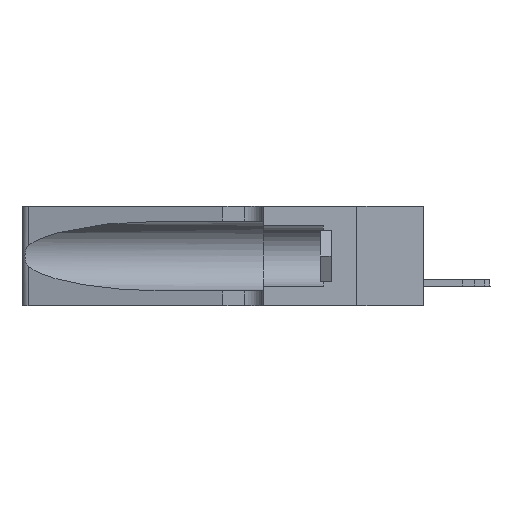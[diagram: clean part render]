
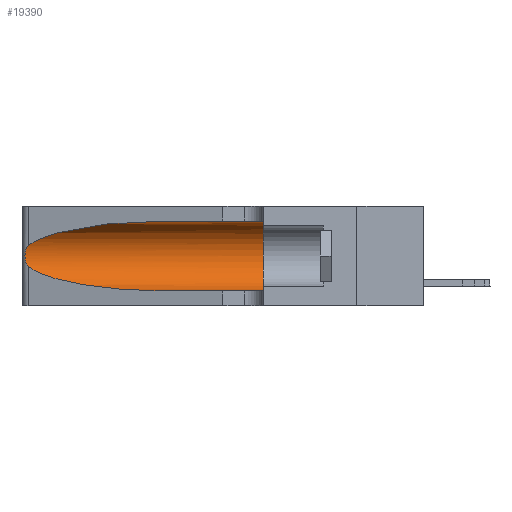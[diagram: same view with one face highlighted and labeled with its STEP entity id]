
A CAD part, left-side view. The second image highlights one B-rep face of the part: STEP entity #19390.
In plain terms, the highlighted cylindrical face has radius 3.308 mm (diameter 6.617 mm), a partial arc.
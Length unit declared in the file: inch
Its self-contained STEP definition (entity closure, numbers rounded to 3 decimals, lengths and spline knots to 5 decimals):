
#1160 = EDGE_CURVE ( 'NONE', #10669, #20331, #22495, .T. ) ;
#1210 = CARTESIAN_POINT ( 'NONE',  ( 0.25487, 1.22718, 0.22369 ) ) ;
#1453 = VERTEX_POINT ( 'NONE', #5880 ) ;
#1458 = AXIS2_PLACEMENT_3D ( 'NONE', #6180, #21093, #14717 ) ;
#3274 = CARTESIAN_POINT ( 'NONE',  ( 0.1305, 1.61858, 0.31525 ) ) ;
#3542 = CARTESIAN_POINT ( 'NONE',  ( 0.1305, 1.61858, 0.05475 ) ) ;
#3585 =( BOUNDED_CURVE ( )  B_SPLINE_CURVE ( 3, ( #24011, #21808, #19467, #15266 ),
 .UNSPECIFIED., .F., .F. ) 
 B_SPLINE_CURVE_WITH_KNOTS ( ( 4, 4 ),
 ( 3.44316, 4.71239 ),
 .UNSPECIFIED. ) 
 CURVE ( )  GEOMETRIC_REPRESENTATION_ITEM ( )  RATIONAL_B_SPLINE_CURVE ( ( 1., 0.87, 0.87, 1. ) ) 
 REPRESENTATION_ITEM ( '' )  );
#4098 = CYLINDRICAL_SURFACE ( 'NONE', #4486, 0.13025 ) ;
#4153 = LINE ( 'NONE', #3274, #22748 ) ;
#4486 = AXIS2_PLACEMENT_3D ( 'NONE', #14302, #27148, #7990 ) ;
#4763 = FACE_OUTER_BOUND ( 'NONE', #14168, .T. ) ;
#4936 = CARTESIAN_POINT ( 'NONE',  ( 0.1305, 0.72297, 0.31525 ) ) ;
#5878 = CARTESIAN_POINT ( 'NONE',  ( 0.26075, 1.23896, 0.178 ) ) ;
#5880 = CARTESIAN_POINT ( 'NONE',  ( 0.1305, 0.35, 0.05475 ) ) ;
#5947 = B_SPLINE_CURVE_WITH_KNOTS ( 'NONE', 3,
 ( #18509, #6045, #10028, #24920, #16462, #18599, #12280, #5878, #20768, #12462, #10219, #12368, #20968, #7999 ),
 .UNSPECIFIED., .F., .F.,
 ( 4, 2, 2, 2, 2, 2, 4 ),
 ( 0., 0.00027, 0.00053, 0.00107, 0.0016, 0.00187, 0.00214 ),
 .UNSPECIFIED. ) ;
#6045 = CARTESIAN_POINT ( 'NONE',  ( 0.25555, 1.22994, 0.2215 ) ) ;
#6071 = ORIENTED_EDGE ( 'NONE', *, *, #1160, .T. ) ;
#6139 = CARTESIAN_POINT ( 'NONE',  ( 0.1305, 0.35, 0.31525 ) ) ;
#6180 = CARTESIAN_POINT ( 'NONE',  ( 0.1305, 0.35, 0.185 ) ) ;
#7990 = DIRECTION ( 'NONE',  ( 0., 0., -1. ) ) ;
#7999 = CARTESIAN_POINT ( 'NONE',  ( 0.25487, 1.22718, 0.14631 ) ) ;
#8107 = CARTESIAN_POINT ( 'NONE',  ( 0.18966, 0.96281, 0.31525 ) ) ;
#8493 = ORIENTED_EDGE ( 'NONE', *, *, #20028, .T. ) ;
#9845 = ORIENTED_EDGE ( 'NONE', *, *, #16774, .T. ) ;
#10028 = CARTESIAN_POINT ( 'NONE',  ( 0.25639, 1.23184, 0.21858 ) ) ;
#10219 = CARTESIAN_POINT ( 'NONE',  ( 0.25789, 1.23486, 0.15765 ) ) ;
#10669 = VERTEX_POINT ( 'NONE', #4936 ) ;
#11089 = VERTEX_POINT ( 'NONE', #26609 ) ;
#11314 = VERTEX_POINT ( 'NONE', #6139 ) ;
#11347 = ORIENTED_EDGE ( 'NONE', *, *, #13831, .T. ) ;
#12111 = VERTEX_POINT ( 'NONE', #17732 ) ;
#12280 = CARTESIAN_POINT ( 'NONE',  ( 0.26075, 1.23896, 0.19203 ) ) ;
#12368 = CARTESIAN_POINT ( 'NONE',  ( 0.25639, 1.23186, 0.15144 ) ) ;
#12462 = CARTESIAN_POINT ( 'NONE',  ( 0.25856, 1.23593, 0.16098 ) ) ;
#13447 = EDGE_CURVE ( 'NONE', #10669, #11314, #4153, .T. ) ;
#13667 = VECTOR ( 'NONE', #24621, 39.37008 ) ;
#13831 = EDGE_CURVE ( 'NONE', #11089, #12111, #3585, .T. ) ;
#14168 = EDGE_LOOP ( 'NONE', ( #6071, #9845, #11347, #8493, #18073, #17289 ) ) ;
#14302 = CARTESIAN_POINT ( 'NONE',  ( 0.1305, 1.61858, 0.185 ) ) ;
#14717 = DIRECTION ( 'NONE',  ( 0., 0., 1. ) ) ;
#15266 = CARTESIAN_POINT ( 'NONE',  ( 0.1305, 0.72297, 0.05475 ) ) ;
#16253 = EDGE_CURVE ( 'NONE', #11314, #1453, #23301, .T. ) ;
#16462 = CARTESIAN_POINT ( 'NONE',  ( 0.25854, 1.2359, 0.20912 ) ) ;
#16753 = CARTESIAN_POINT ( 'NONE',  ( 0.2373, 1.15595, 0.28018 ) ) ;
#16774 = EDGE_CURVE ( 'NONE', #20331, #11089, #5947, .T. ) ;
#17289 = ORIENTED_EDGE ( 'NONE', *, *, #13447, .F. ) ;
#17732 = CARTESIAN_POINT ( 'NONE',  ( 0.1305, 0.72297, 0.05475 ) ) ;
#17854 = DIRECTION ( 'NONE',  ( 0., -1., 0. ) ) ;
#18073 = ORIENTED_EDGE ( 'NONE', *, *, #16253, .F. ) ;
#18509 = CARTESIAN_POINT ( 'NONE',  ( 0.25487, 1.22718, 0.22369 ) ) ;
#18599 = CARTESIAN_POINT ( 'NONE',  ( 0.26018, 1.23835, 0.19895 ) ) ;
#19390 = ADVANCED_FACE ( 'NONE', ( #4763 ), #4098, .F. ) ;
#19467 = CARTESIAN_POINT ( 'NONE',  ( 0.18966, 0.96281, 0.05475 ) ) ;
#20019 = LINE ( 'NONE', #3542, #13667 ) ;
#20028 = EDGE_CURVE ( 'NONE', #12111, #1453, #20019, .T. ) ;
#20331 = VERTEX_POINT ( 'NONE', #1210 ) ;
#20768 = CARTESIAN_POINT ( 'NONE',  ( 0.26017, 1.23833, 0.17102 ) ) ;
#20887 = CARTESIAN_POINT ( 'NONE',  ( 0.1305, 0.72297, 0.31525 ) ) ;
#20968 = CARTESIAN_POINT ( 'NONE',  ( 0.25555, 1.22993, 0.14849 ) ) ;
#21093 = DIRECTION ( 'NONE',  ( 0., 1., 0. ) ) ;
#21808 = CARTESIAN_POINT ( 'NONE',  ( 0.2373, 1.15595, 0.08982 ) ) ;
#22495 =( BOUNDED_CURVE ( )  B_SPLINE_CURVE ( 3, ( #20887, #8107, #16753, #22994 ),
 .UNSPECIFIED., .F., .F. ) 
 B_SPLINE_CURVE_WITH_KNOTS ( ( 4, 4 ),
 ( 1.5708, 2.84003 ),
 .UNSPECIFIED. ) 
 CURVE ( )  GEOMETRIC_REPRESENTATION_ITEM ( )  RATIONAL_B_SPLINE_CURVE ( ( 1., 0.87, 0.87, 1. ) ) 
 REPRESENTATION_ITEM ( '' )  );
#22748 = VECTOR ( 'NONE', #17854, 39.37008 ) ;
#22994 = CARTESIAN_POINT ( 'NONE',  ( 0.25487, 1.22718, 0.22369 ) ) ;
#23301 = CIRCLE ( 'NONE', #1458, 0.13025 ) ;
#24011 = CARTESIAN_POINT ( 'NONE',  ( 0.25487, 1.22718, 0.14631 ) ) ;
#24621 = DIRECTION ( 'NONE',  ( 0., -1., 0. ) ) ;
#24920 = CARTESIAN_POINT ( 'NONE',  ( 0.25787, 1.23484, 0.2124 ) ) ;
#26609 = CARTESIAN_POINT ( 'NONE',  ( 0.25487, 1.22718, 0.14631 ) ) ;
#27148 = DIRECTION ( 'NONE',  ( 0., -1., 0. ) ) ;
